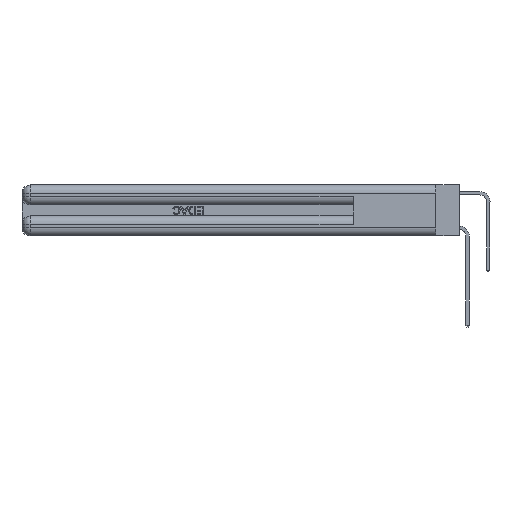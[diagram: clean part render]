
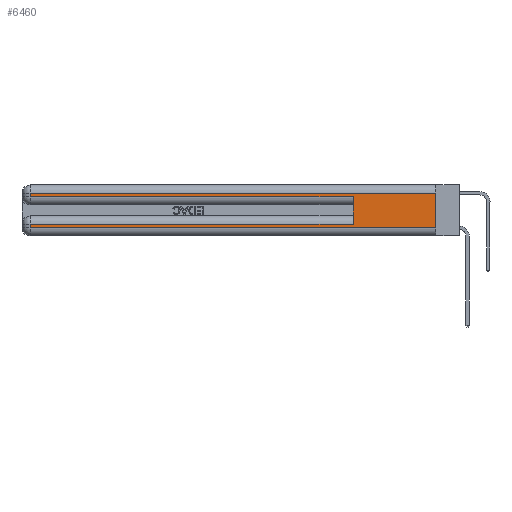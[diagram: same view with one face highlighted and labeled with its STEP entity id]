
A CAD part, left-side view. The second image highlights one B-rep face of the part: STEP entity #6460.
In plain terms, the highlighted planar face has unit normal (-1, 0, 0).
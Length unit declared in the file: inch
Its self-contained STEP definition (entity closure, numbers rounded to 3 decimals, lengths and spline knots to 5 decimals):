
#869 = LINE ( 'NONE', #5610, #19695 ) ;
#925 = VERTEX_POINT ( 'NONE', #1576 ) ;
#1049 = ORIENTED_EDGE ( 'NONE', *, *, #4378, .F. ) ;
#1158 = CARTESIAN_POINT ( 'NONE',  ( 0., 0., 0.085 ) ) ;
#1195 = DIRECTION ( 'NONE',  ( 0., 0., -1. ) ) ;
#1272 = VERTEX_POINT ( 'NONE', #16899 ) ;
#1576 = CARTESIAN_POINT ( 'NONE',  ( 0., 2.94, 0.31 ) ) ;
#1934 = DIRECTION ( 'NONE',  ( 1., 0., 0. ) ) ;
#1991 = CARTESIAN_POINT ( 'NONE',  ( 0., 0., 0.37 ) ) ;
#2354 = CARTESIAN_POINT ( 'NONE',  ( 0., 2.94, 0.37 ) ) ;
#2728 = CARTESIAN_POINT ( 'NONE',  ( 0., 0., 0.06 ) ) ;
#2762 = EDGE_CURVE ( 'NONE', #6031, #32368, #5732, .T. ) ;
#3683 = LINE ( 'NONE', #1991, #31470 ) ;
#3840 = ORIENTED_EDGE ( 'NONE', *, *, #22575, .T. ) ;
#4360 = VECTOR ( 'NONE', #31505, 39.37008 ) ;
#4378 = EDGE_CURVE ( 'NONE', #1272, #15194, #3683, .T. ) ;
#5610 = CARTESIAN_POINT ( 'NONE',  ( 0., 0., 0.31 ) ) ;
#5732 = LINE ( 'NONE', #30699, #15500 ) ;
#6031 = VERTEX_POINT ( 'NONE', #18043 ) ;
#6460 = ADVANCED_FACE ( 'NONE', ( #23896 ), #11846, .F. ) ;
#6904 = VECTOR ( 'NONE', #1195, 39.37008 ) ;
#7881 = CARTESIAN_POINT ( 'NONE',  ( 0., 0.6, 0.285 ) ) ;
#9024 = VECTOR ( 'NONE', #29608, 39.37008 ) ;
#9040 = CARTESIAN_POINT ( 'NONE',  ( 0., 0., 0.06 ) ) ;
#9449 = DIRECTION ( 'NONE',  ( 0., 0., -1. ) ) ;
#11226 = LINE ( 'NONE', #18777, #14740 ) ;
#11730 = EDGE_CURVE ( 'NONE', #32470, #20849, #26881, .T. ) ;
#11772 = LINE ( 'NONE', #9040, #4360 ) ;
#11846 = PLANE ( 'NONE',  #21624 ) ;
#12848 = CARTESIAN_POINT ( 'NONE',  ( 0., 2.94, 0.285 ) ) ;
#14354 = CARTESIAN_POINT ( 'NONE',  ( 0., 0., 0.37 ) ) ;
#14740 = VECTOR ( 'NONE', #29614, 39.37008 ) ;
#15011 = ORIENTED_EDGE ( 'NONE', *, *, #24330, .T. ) ;
#15194 = VERTEX_POINT ( 'NONE', #2728 ) ;
#15193 = ORIENTED_EDGE ( 'NONE', *, *, #11730, .T. ) ;
#15500 = VECTOR ( 'NONE', #23211, 39.37008 ) ;
#16558 = ORIENTED_EDGE ( 'NONE', *, *, #16729, .T. ) ;
#16729 = EDGE_CURVE ( 'NONE', #6031, #32470, #31843, .T. ) ;
#16899 = CARTESIAN_POINT ( 'NONE',  ( 0., 0., 0.31 ) ) ;
#17233 = ORIENTED_EDGE ( 'NONE', *, *, #2762, .F. ) ;
#18043 = CARTESIAN_POINT ( 'NONE',  ( 0., 0.6, 0.085 ) ) ;
#18302 = CARTESIAN_POINT ( 'NONE',  ( 0., 2.94, 0.085 ) ) ;
#18488 = CARTESIAN_POINT ( 'NONE',  ( 0., 2.94, 0.37 ) ) ;
#18777 = CARTESIAN_POINT ( 'NONE',  ( 0., 0., 0.285 ) ) ;
#19695 = VECTOR ( 'NONE', #30804, 39.37008 ) ;
#19721 = EDGE_LOOP ( 'NONE', ( #1049, #32104, #3840, #15011, #17233, #16558, #15193, #24181 ) ) ;
#20849 = VERTEX_POINT ( 'NONE', #31076 ) ;
#21216 = VECTOR ( 'NONE', #31380, 39.37008 ) ;
#21624 = AXIS2_PLACEMENT_3D ( 'NONE', #14354, #1934, #9449 ) ;
#22575 = EDGE_CURVE ( 'NONE', #925, #29891, #27064, .T. ) ;
#23211 = DIRECTION ( 'NONE',  ( 0., 0., 1. ) ) ;
#23896 = FACE_OUTER_BOUND ( 'NONE', #19721, .T. ) ;
#24181 = ORIENTED_EDGE ( 'NONE', *, *, #31365, .T. ) ;
#24330 = EDGE_CURVE ( 'NONE', #29891, #32368, #11226, .T. ) ;
#24655 = DIRECTION ( 'NONE',  ( 0., 0., -1. ) ) ;
#26881 = LINE ( 'NONE', #18488, #6904 ) ;
#27064 = LINE ( 'NONE', #2354, #9024 ) ;
#29608 = DIRECTION ( 'NONE',  ( 0., 0., -1. ) ) ;
#29614 = DIRECTION ( 'NONE',  ( 0., -1., 0. ) ) ;
#29891 = VERTEX_POINT ( 'NONE', #12848 ) ;
#30571 = EDGE_CURVE ( 'NONE', #1272, #925, #869, .T. ) ;
#30699 = CARTESIAN_POINT ( 'NONE',  ( 0., 0.6, 0.145 ) ) ;
#30804 = DIRECTION ( 'NONE',  ( 0., 1., 0. ) ) ;
#31076 = CARTESIAN_POINT ( 'NONE',  ( 0., 2.94, 0.06 ) ) ;
#31365 = EDGE_CURVE ( 'NONE', #20849, #15194, #11772, .T. ) ;
#31380 = DIRECTION ( 'NONE',  ( 0., 1., 0. ) ) ;
#31470 = VECTOR ( 'NONE', #24655, 39.37008 ) ;
#31505 = DIRECTION ( 'NONE',  ( 0., -1., 0. ) ) ;
#31843 = LINE ( 'NONE', #1158, #21216 ) ;
#32104 = ORIENTED_EDGE ( 'NONE', *, *, #30571, .T. ) ;
#32368 = VERTEX_POINT ( 'NONE', #7881 ) ;
#32470 = VERTEX_POINT ( 'NONE', #18302 ) ;
